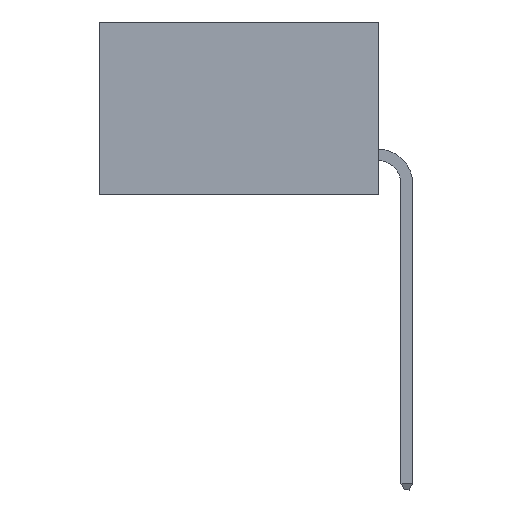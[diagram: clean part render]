
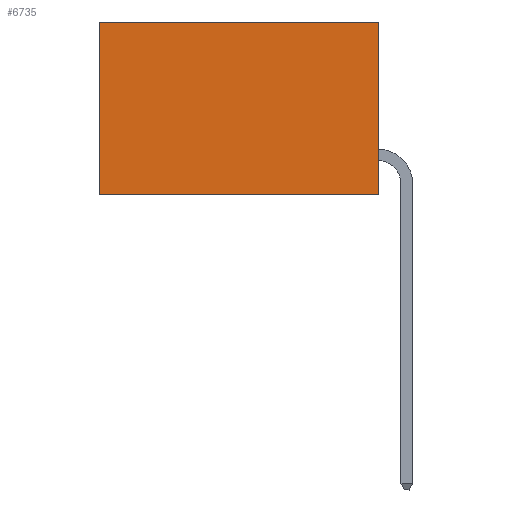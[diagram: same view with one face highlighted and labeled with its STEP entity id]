
A CAD part, left-side view. The second image highlights one B-rep face of the part: STEP entity #6735.
In plain terms, the highlighted planar face has unit normal (-1, 0, 0).
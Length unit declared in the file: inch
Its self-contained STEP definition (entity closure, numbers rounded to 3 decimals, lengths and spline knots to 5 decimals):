
#707 = CARTESIAN_POINT ( 'NONE',  ( 0.298, 0., 0. ) ) ;
#728 = EDGE_CURVE ( 'NONE', #4575, #9595, #1780, .T. ) ;
#730 = ORIENTED_EDGE ( 'NONE', *, *, #728, .T. ) ;
#878 = CARTESIAN_POINT ( 'NONE',  ( 0.298, 0., 0. ) ) ;
#1177 = ORIENTED_EDGE ( 'NONE', *, *, #6798, .F. ) ;
#1549 = CARTESIAN_POINT ( 'NONE',  ( 0.298, 0., 0. ) ) ;
#1617 = VERTEX_POINT ( 'NONE', #9816 ) ;
#1780 = LINE ( 'NONE', #878, #2036 ) ;
#2036 = VECTOR ( 'NONE', #7028, 39.37008 ) ;
#2578 = CARTESIAN_POINT ( 'NONE',  ( 0.298, 0.6, 0. ) ) ;
#2598 = CARTESIAN_POINT ( 'NONE',  ( 0.298, 0., -0.37 ) ) ;
#2658 = DIRECTION ( 'NONE',  ( 0., 0., -1. ) ) ;
#3449 = CARTESIAN_POINT ( 'NONE',  ( 0.298, 0., 0. ) ) ;
#4575 = VERTEX_POINT ( 'NONE', #3449 ) ;
#4908 = EDGE_CURVE ( 'NONE', #1617, #10906, #10394, .T. ) ;
#4997 = VECTOR ( 'NONE', #2658, 39.37008 ) ;
#5005 = AXIS2_PLACEMENT_3D ( 'NONE', #1549, #7709, #10273 ) ;
#5935 = CARTESIAN_POINT ( 'NONE',  ( 0.298, 0.6, 0. ) ) ;
#5955 = LINE ( 'NONE', #707, #4997 ) ;
#6197 = DIRECTION ( 'NONE',  ( 0., 1., 0. ) ) ;
#6709 = DIRECTION ( 'NONE',  ( 0., 0., -1. ) ) ;
#6735 = ADVANCED_FACE ( 'NONE', ( #6933 ), #9499, .F. ) ;
#6798 = EDGE_CURVE ( 'NONE', #4575, #1617, #5955, .T. ) ;
#6933 = FACE_OUTER_BOUND ( 'NONE', #8447, .T. ) ;
#7028 = DIRECTION ( 'NONE',  ( 0., 1., 0. ) ) ;
#7282 = LINE ( 'NONE', #5935, #9352 ) ;
#7709 = DIRECTION ( 'NONE',  ( 1., 0., 0. ) ) ;
#7936 = VECTOR ( 'NONE', #6197, 39.37008 ) ;
#8447 = EDGE_LOOP ( 'NONE', ( #9378, #10464, #1177, #730 ) ) ;
#9352 = VECTOR ( 'NONE', #6709, 39.37008 ) ;
#9378 = ORIENTED_EDGE ( 'NONE', *, *, #10482, .T. ) ;
#9499 = PLANE ( 'NONE',  #5005 ) ;
#9595 = VERTEX_POINT ( 'NONE', #2578 ) ;
#9802 = CARTESIAN_POINT ( 'NONE',  ( 0.298, 0.6, -0.37 ) ) ;
#9816 = CARTESIAN_POINT ( 'NONE',  ( 0.298, 0., -0.37 ) ) ;
#10273 = DIRECTION ( 'NONE',  ( 0., 0., -1. ) ) ;
#10394 = LINE ( 'NONE', #2598, #7936 ) ;
#10464 = ORIENTED_EDGE ( 'NONE', *, *, #4908, .F. ) ;
#10482 = EDGE_CURVE ( 'NONE', #9595, #10906, #7282, .T. ) ;
#10906 = VERTEX_POINT ( 'NONE', #9802 ) ;
